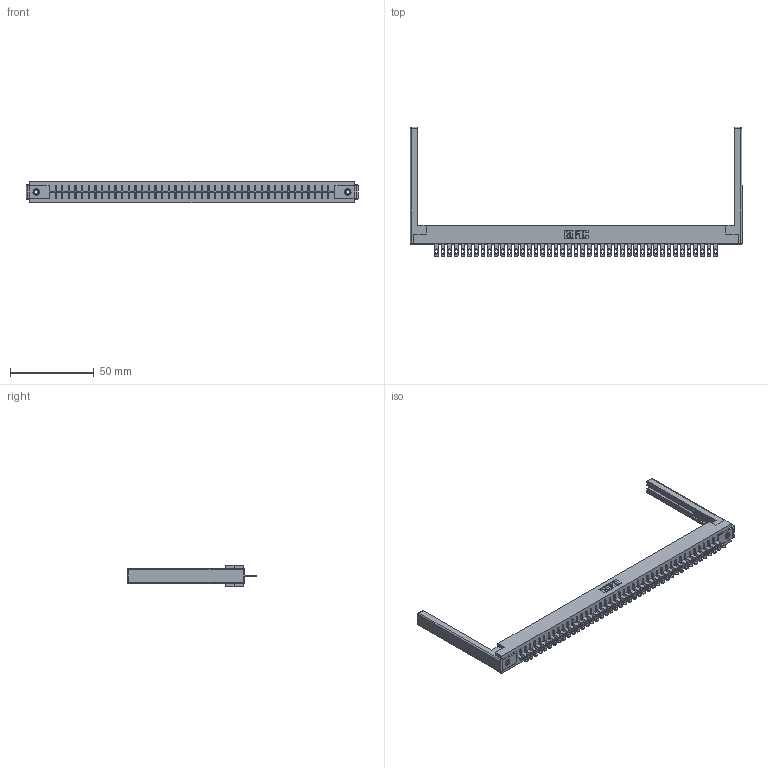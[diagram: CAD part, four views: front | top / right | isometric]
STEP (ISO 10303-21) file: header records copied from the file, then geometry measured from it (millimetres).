
FILE_DESCRIPTION (( 'STEP AP203' ), '1' );
FILE_NAME ('316-043-500-168.STEP', '2018-07-31T05:58:59', ( '' ), ( '' ), 'SwSTEP 2.0', 'SolidWorks 2016', '' );
FILE_SCHEMA (( 'CONFIG_CONTROL_DESIGN' ));
Length unit declared in the file: inch
Products named in the file (5): 306 Part_.156 Dia; 306-290-001_100; 345-250-001_345-250-001-102; 307-220-068; 316-043-500-168
Assembly tree (48 placements, depth 2):
  316-043-500-168
    306 Part_.156 Dia
    306-290-001_100  x43
    345-250-001_345-250-001-102  x2
    307-220-068  x2
Bounding box: 197.82 x 77.17 x 12.7 mm (x, y, z)
Volume: 26393.9 mm3; surface area: 27428.5 mm2
Topology: 48 solids, 48 shells, 3538 faces, 9951 edges, 6382 vertices
Faces by surface type: plane 2306, cylinder 1036, sphere 180, cone 12, torus 4
Entity records: 42893 total; most frequent: CARTESIAN_POINT 7169, ORIENTED_EDGE 7100, DIRECTION 7082, EDGE_CURVE 3550, VECTOR 2772, LINE 2772, VERTEX_POINT 2242, AXIS2_PLACEMENT_3D 2155
